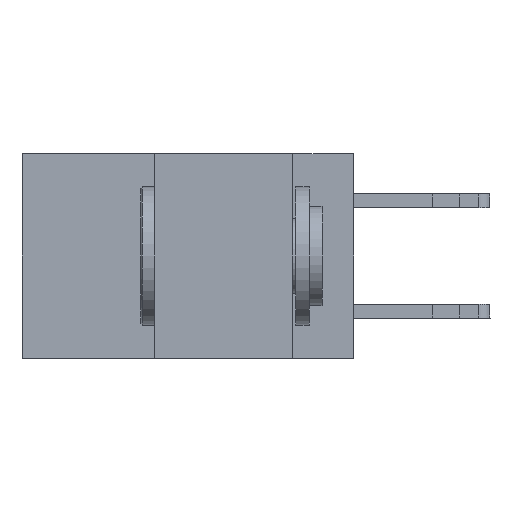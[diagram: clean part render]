
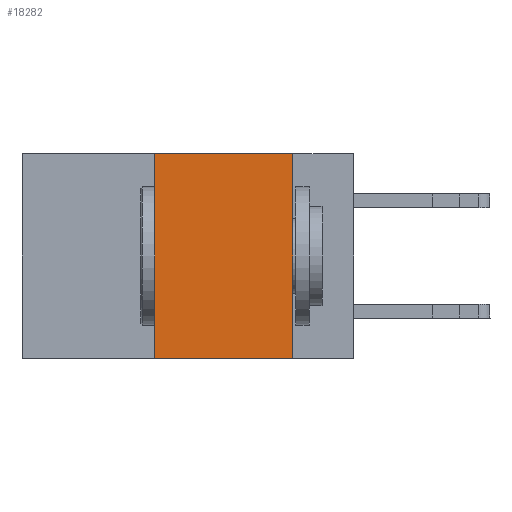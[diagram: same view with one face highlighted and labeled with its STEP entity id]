
A CAD part, left-side view. The second image highlights one B-rep face of the part: STEP entity #18282.
In plain terms, the highlighted planar face has unit normal (-1, 0, 0).
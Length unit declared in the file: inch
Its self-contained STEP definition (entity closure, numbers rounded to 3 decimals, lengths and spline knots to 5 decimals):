
#1144 = ORIENTED_EDGE ( 'NONE', *, *, #11147, .T. ) ;
#2589 = ORIENTED_EDGE ( 'NONE', *, *, #20609, .F. ) ;
#3661 = CARTESIAN_POINT ( 'NONE',  ( 0., 0.6, -0.37 ) ) ;
#3686 = VECTOR ( 'NONE', #11630, 39.37008 ) ;
#4738 = VERTEX_POINT ( 'NONE', #17431 ) ;
#4745 = CARTESIAN_POINT ( 'NONE',  ( 0., 0.36, 0. ) ) ;
#5165 = PLANE ( 'NONE',  #23053 ) ;
#5952 = EDGE_LOOP ( 'NONE', ( #2589, #7447, #14473, #1144 ) ) ;
#6149 = VERTEX_POINT ( 'NONE', #23147 ) ;
#6163 = CARTESIAN_POINT ( 'NONE',  ( 0., 0.11, 0. ) ) ;
#6312 = EDGE_CURVE ( 'NONE', #4738, #6616, #8451, .T. ) ;
#6616 = VERTEX_POINT ( 'NONE', #20962 ) ;
#7021 = DIRECTION ( 'NONE',  ( 1., 0., 0. ) ) ;
#7447 = ORIENTED_EDGE ( 'NONE', *, *, #6312, .F. ) ;
#8451 = LINE ( 'NONE', #21879, #17325 ) ;
#9402 = LINE ( 'NONE', #4745, #18252 ) ;
#9469 = EDGE_CURVE ( 'NONE', #6149, #4738, #9402, .T. ) ;
#10412 = VERTEX_POINT ( 'NONE', #18082 ) ;
#11147 = EDGE_CURVE ( 'NONE', #6149, #10412, #20389, .T. ) ;
#11630 = DIRECTION ( 'NONE',  ( 0., 0., -1. ) ) ;
#12043 = DIRECTION ( 'NONE',  ( 0., 0., 1. ) ) ;
#12847 = DIRECTION ( 'NONE',  ( 0., -1., 0. ) ) ;
#13112 = FACE_OUTER_BOUND ( 'NONE', #5952, .T. ) ;
#14473 = ORIENTED_EDGE ( 'NONE', *, *, #9469, .F. ) ;
#14917 = DIRECTION ( 'NONE',  ( 0., -1., 0. ) ) ;
#15723 = VECTOR ( 'NONE', #12847, 39.37008 ) ;
#15868 = CARTESIAN_POINT ( 'NONE',  ( 0., 0.6, 0. ) ) ;
#17325 = VECTOR ( 'NONE', #14917, 39.37008 ) ;
#17410 = LINE ( 'NONE', #6163, #3686 ) ;
#17431 = CARTESIAN_POINT ( 'NONE',  ( 0., 0.36, 0. ) ) ;
#18082 = CARTESIAN_POINT ( 'NONE',  ( 0., 0.11, -0.37 ) ) ;
#18252 = VECTOR ( 'NONE', #12043, 39.37008 ) ;
#18282 = ADVANCED_FACE ( 'NONE', ( #13112 ), #5165, .F. ) ;
#19438 = DIRECTION ( 'NONE',  ( 0., 0., -1. ) ) ;
#20389 = LINE ( 'NONE', #3661, #15723 ) ;
#20609 = EDGE_CURVE ( 'NONE', #6616, #10412, #17410, .T. ) ;
#20962 = CARTESIAN_POINT ( 'NONE',  ( 0., 0.11, 0. ) ) ;
#21879 = CARTESIAN_POINT ( 'NONE',  ( 0., 0.6, 0. ) ) ;
#23053 = AXIS2_PLACEMENT_3D ( 'NONE', #15868, #7021, #19438 ) ;
#23147 = CARTESIAN_POINT ( 'NONE',  ( 0., 0.36, -0.37 ) ) ;
